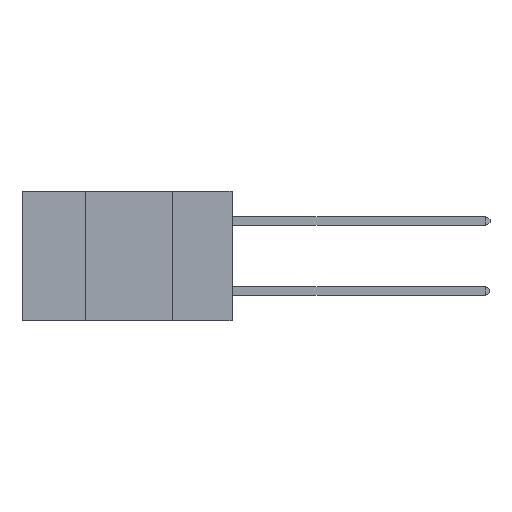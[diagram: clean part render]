
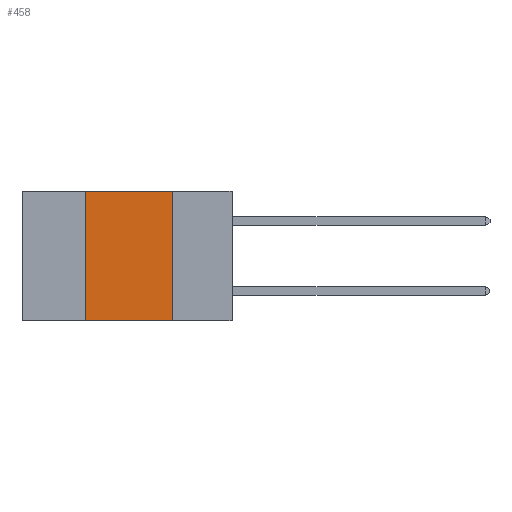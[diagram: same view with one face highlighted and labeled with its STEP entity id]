
A CAD part, left-side view. The second image highlights one B-rep face of the part: STEP entity #458.
In plain terms, the highlighted planar face has unit normal (-1, 0, 0).
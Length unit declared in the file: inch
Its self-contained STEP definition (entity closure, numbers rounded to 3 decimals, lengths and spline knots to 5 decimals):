
#458 = ADVANCED_FACE ( 'NONE', ( #7585 ), #23051, .F. ) ;
#659 = VERTEX_POINT ( 'NONE', #11551 ) ;
#1131 = LINE ( 'NONE', #19262, #14852 ) ;
#1387 = CARTESIAN_POINT ( 'NONE',  ( 0., 0.42, 0. ) ) ;
#2343 = EDGE_CURVE ( 'NONE', #659, #7586, #1131, .T. ) ;
#2883 = VERTEX_POINT ( 'NONE', #10131 ) ;
#5108 = EDGE_CURVE ( 'NONE', #2883, #17675, #21801, .T. ) ;
#5301 = EDGE_CURVE ( 'NONE', #17675, #659, #9559, .T. ) ;
#5316 = ORIENTED_EDGE ( 'NONE', *, *, #2343, .F. ) ;
#6260 = CARTESIAN_POINT ( 'NONE',  ( 0., 0.17, -0.37 ) ) ;
#6734 = VECTOR ( 'NONE', #16017, 39.37008 ) ;
#7540 = DIRECTION ( 'NONE',  ( 0., -1., 0. ) ) ;
#7585 = FACE_OUTER_BOUND ( 'NONE', #22459, .T. ) ;
#7586 = VERTEX_POINT ( 'NONE', #6260 ) ;
#7923 = LINE ( 'NONE', #23113, #6734 ) ;
#9173 = DIRECTION ( 'NONE',  ( 0., 0., 1. ) ) ;
#9442 = EDGE_CURVE ( 'NONE', #2883, #7586, #7923, .T. ) ;
#9559 = LINE ( 'NONE', #12978, #22649 ) ;
#10131 = CARTESIAN_POINT ( 'NONE',  ( 0., 0.42, -0.37 ) ) ;
#10162 = ORIENTED_EDGE ( 'NONE', *, *, #9442, .T. ) ;
#11551 = CARTESIAN_POINT ( 'NONE',  ( 0., 0.17, 0. ) ) ;
#12978 = CARTESIAN_POINT ( 'NONE',  ( 0., 0.6, 0. ) ) ;
#14846 = ORIENTED_EDGE ( 'NONE', *, *, #5301, .F. ) ;
#14852 = VECTOR ( 'NONE', #15739, 39.37008 ) ;
#15177 = AXIS2_PLACEMENT_3D ( 'NONE', #22405, #15411, #16961 ) ;
#15411 = DIRECTION ( 'NONE',  ( 1., 0., 0. ) ) ;
#15739 = DIRECTION ( 'NONE',  ( 0., 0., -1. ) ) ;
#16017 = DIRECTION ( 'NONE',  ( 0., -1., 0. ) ) ;
#16776 = ORIENTED_EDGE ( 'NONE', *, *, #5108, .F. ) ;
#16961 = DIRECTION ( 'NONE',  ( 0., 0., -1. ) ) ;
#17149 = CARTESIAN_POINT ( 'NONE',  ( 0., 0.42, 0. ) ) ;
#17675 = VERTEX_POINT ( 'NONE', #17149 ) ;
#19262 = CARTESIAN_POINT ( 'NONE',  ( 0., 0.17, 0. ) ) ;
#21280 = VECTOR ( 'NONE', #9173, 39.37008 ) ;
#21801 = LINE ( 'NONE', #1387, #21280 ) ;
#22405 = CARTESIAN_POINT ( 'NONE',  ( 0., 0.6, 0. ) ) ;
#22459 = EDGE_LOOP ( 'NONE', ( #5316, #14846, #16776, #10162 ) ) ;
#22649 = VECTOR ( 'NONE', #7540, 39.37008 ) ;
#23051 = PLANE ( 'NONE',  #15177 ) ;
#23113 = CARTESIAN_POINT ( 'NONE',  ( 0., 0.6, -0.37 ) ) ;
